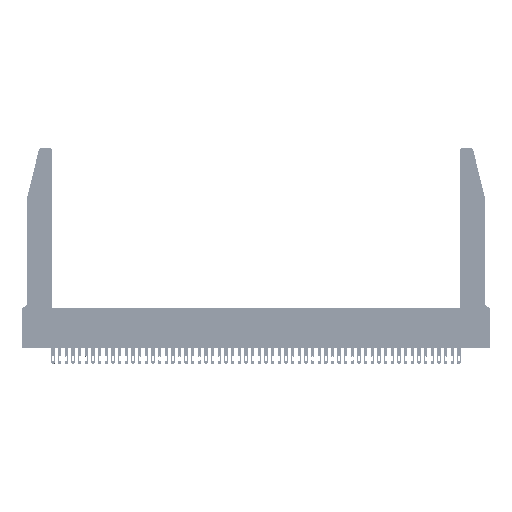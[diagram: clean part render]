
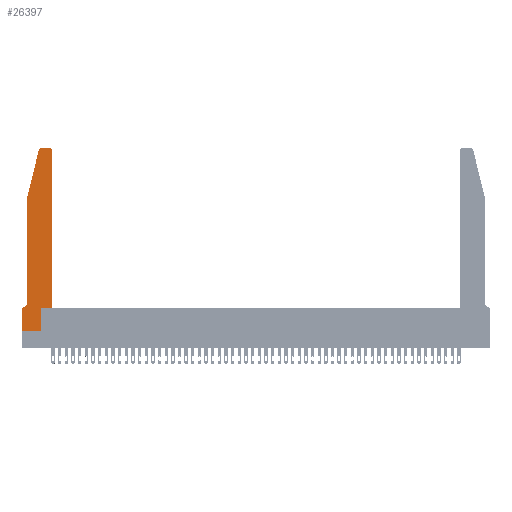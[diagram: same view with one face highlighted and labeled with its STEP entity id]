
A CAD part, top view. The second image highlights one B-rep face of the part: STEP entity #26397.
In plain terms, the highlighted planar face has unit normal (0, 0, 1).
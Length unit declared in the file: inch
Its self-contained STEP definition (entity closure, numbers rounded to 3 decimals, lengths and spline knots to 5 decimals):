
#550 = DIRECTION ( 'NONE',  ( -1., 0., 0. ) ) ;
#915 = CARTESIAN_POINT ( 'NONE',  ( 0.4505, 0.35, 0.37 ) ) ;
#1173 = VECTOR ( 'NONE', #18549, 39.37008 ) ;
#1265 = LINE ( 'NONE', #35917, #48980 ) ;
#2085 = AXIS2_PLACEMENT_3D ( 'NONE', #5946, #13271, #40658 ) ;
#2260 = ORIENTED_EDGE ( 'NONE', *, *, #8568, .T. ) ;
#3101 = DIRECTION ( 'NONE',  ( 1., 0., 0. ) ) ;
#3153 = EDGE_CURVE ( 'NONE', #23213, #50517, #5356, .T. ) ;
#3368 = CARTESIAN_POINT ( 'NONE',  ( 0., 0.35, 0.37 ) ) ;
#3682 = ORIENTED_EDGE ( 'NONE', *, *, #30100, .T. ) ;
#5268 = VECTOR ( 'NONE', #24191, 39.37008 ) ;
#5356 = LINE ( 'NONE', #44972, #32894 ) ;
#5617 = CARTESIAN_POINT ( 'NONE',  ( 0.4505, 0.35, 0.37 ) ) ;
#5848 = LINE ( 'NONE', #27617, #5268 ) ;
#5946 = CARTESIAN_POINT ( 'NONE',  ( 0.0055, 0.42, 0.37 ) ) ;
#6176 = VERTEX_POINT ( 'NONE', #3368 ) ;
#7727 = LINE ( 'NONE', #30731, #32263 ) ;
#8096 = CARTESIAN_POINT ( 'NONE',  ( 0.0755, 0.35, 0.37 ) ) ;
#8448 = EDGE_CURVE ( 'NONE', #16313, #36084, #45249, .T. ) ;
#8568 = EDGE_CURVE ( 'NONE', #17694, #30529, #43979, .T. ) ;
#8913 = ORIENTED_EDGE ( 'NONE', *, *, #10560, .T. ) ;
#8957 = AXIS2_PLACEMENT_3D ( 'NONE', #18659, #46000, #3101 ) ;
#9064 = ORIENTED_EDGE ( 'NONE', *, *, #30528, .T. ) ;
#9164 = LINE ( 'NONE', #34760, #10995 ) ;
#9933 = ORIENTED_EDGE ( 'NONE', *, *, #42092, .T. ) ;
#10155 = ORIENTED_EDGE ( 'NONE', *, *, #8448, .T. ) ;
#10560 = EDGE_CURVE ( 'NONE', #36084, #19034, #23695, .T. ) ;
#10995 = VECTOR ( 'NONE', #35103, 39.37008 ) ;
#11185 = FACE_OUTER_BOUND ( 'NONE', #21468, .T. ) ;
#11554 = VERTEX_POINT ( 'NONE', #20644 ) ;
#12856 = CARTESIAN_POINT ( 'NONE',  ( 0.25487, 2.72718, 0.37 ) ) ;
#12894 = CARTESIAN_POINT ( 'NONE',  ( 0.4205, 2.75, 0.37 ) ) ;
#13271 = DIRECTION ( 'NONE',  ( 0., 0., -1. ) ) ;
#13650 = CARTESIAN_POINT ( 'NONE',  ( 0.2865, 0.35, 0.37 ) ) ;
#14009 = EDGE_CURVE ( 'NONE', #11554, #17195, #1265, .T. ) ;
#14400 = ORIENTED_EDGE ( 'NONE', *, *, #14576, .T. ) ;
#14576 = EDGE_CURVE ( 'NONE', #17195, #17694, #9164, .T. ) ;
#14994 = ORIENTED_EDGE ( 'NONE', *, *, #14009, .T. ) ;
#15561 = VERTEX_POINT ( 'NONE', #39977 ) ;
#16313 = VERTEX_POINT ( 'NONE', #12894 ) ;
#16572 = DIRECTION ( 'NONE',  ( 0., 1., 0. ) ) ;
#16661 = DIRECTION ( 'NONE',  ( 0., 1., 0. ) ) ;
#17195 = VERTEX_POINT ( 'NONE', #13650 ) ;
#17450 = DIRECTION ( 'NONE',  ( 0., -1., 0. ) ) ;
#17694 = VERTEX_POINT ( 'NONE', #5617 ) ;
#17739 = DIRECTION ( 'NONE',  ( 1., 0., 0. ) ) ;
#18122 = AXIS2_PLACEMENT_3D ( 'NONE', #33801, #37242, #17739 ) ;
#18549 = DIRECTION ( 'NONE',  ( -1., 0., 0. ) ) ;
#18600 = CARTESIAN_POINT ( 'NONE',  ( 0.284, 2.75, 0.37 ) ) ;
#18659 = CARTESIAN_POINT ( 'NONE',  ( 0.4205, 2.72, 0.37 ) ) ;
#19034 = VERTEX_POINT ( 'NONE', #12856 ) ;
#20644 = CARTESIAN_POINT ( 'NONE',  ( 0.2865, 0., 0.37 ) ) ;
#21468 = EDGE_LOOP ( 'NONE', ( #10155, #8913, #9064, #26012, #30155, #9933, #26757, #3682, #14994, #14400, #2260, #50630 ) ) ;
#22279 = DIRECTION ( 'NONE',  ( 0., 0., 1. ) ) ;
#22285 = DIRECTION ( 'NONE',  ( 1., 0., 0. ) ) ;
#23201 = VECTOR ( 'NONE', #16661, 39.37008 ) ;
#23213 = VERTEX_POINT ( 'NONE', #44004 ) ;
#23695 = CIRCLE ( 'NONE', #18122, 0.03 ) ;
#24191 = DIRECTION ( 'NONE',  ( -0.239, -0.971, 0. ) ) ;
#26012 = ORIENTED_EDGE ( 'NONE', *, *, #3153, .T. ) ;
#26212 = DIRECTION ( 'NONE',  ( 1., 0., 0. ) ) ;
#26397 = ADVANCED_FACE ( 'NONE', ( #11185 ), #41935, .T. ) ;
#26757 = ORIENTED_EDGE ( 'NONE', *, *, #47592, .T. ) ;
#27617 = CARTESIAN_POINT ( 'NONE',  ( 0.0755, 2., 0.37 ) ) ;
#30100 = EDGE_CURVE ( 'NONE', #45808, #11554, #45047, .T. ) ;
#30155 = ORIENTED_EDGE ( 'NONE', *, *, #49687, .T. ) ;
#30528 = EDGE_CURVE ( 'NONE', #19034, #23213, #5848, .T. ) ;
#30529 = VERTEX_POINT ( 'NONE', #31538 ) ;
#30731 = CARTESIAN_POINT ( 'NONE',  ( 0., 0., 0.37 ) ) ;
#31538 = CARTESIAN_POINT ( 'NONE',  ( 0.4505, 2.72, 0.37 ) ) ;
#32263 = VECTOR ( 'NONE', #35010, 39.37008 ) ;
#32894 = VECTOR ( 'NONE', #17450, 39.37008 ) ;
#33801 = CARTESIAN_POINT ( 'NONE',  ( 0.284, 2.72, 0.37 ) ) ;
#34760 = CARTESIAN_POINT ( 'NONE',  ( 0.4505, 0.35, 0.37 ) ) ;
#35010 = DIRECTION ( 'NONE',  ( 0., -1., 0. ) ) ;
#35103 = DIRECTION ( 'NONE',  ( 1., 0., 0. ) ) ;
#35485 = CARTESIAN_POINT ( 'NONE',  ( 0.2605, 2.75, 0.37 ) ) ;
#35917 = CARTESIAN_POINT ( 'NONE',  ( 0.2865, 0.35, 0.37 ) ) ;
#36084 = VERTEX_POINT ( 'NONE', #18600 ) ;
#37242 = DIRECTION ( 'NONE',  ( 0., 0., 1. ) ) ;
#38132 = CIRCLE ( 'NONE', #2085, 0.07 ) ;
#38655 = CARTESIAN_POINT ( 'NONE',  ( 0., 0.35, 0.37 ) ) ;
#39465 = AXIS2_PLACEMENT_3D ( 'NONE', #38655, #22279, #26212 ) ;
#39977 = CARTESIAN_POINT ( 'NONE',  ( 0.0055, 0.35, 0.37 ) ) ;
#40399 = VECTOR ( 'NONE', #550, 39.37008 ) ;
#40658 = DIRECTION ( 'NONE',  ( -1., 0., 0. ) ) ;
#40732 = CARTESIAN_POINT ( 'NONE',  ( 0., 0., 0.37 ) ) ;
#41381 = VECTOR ( 'NONE', #22285, 39.37008 ) ;
#41935 = PLANE ( 'NONE',  #39465 ) ;
#42092 = EDGE_CURVE ( 'NONE', #15561, #6176, #47092, .T. ) ;
#42493 = CARTESIAN_POINT ( 'NONE',  ( 0.0755, 0.42, 0.37 ) ) ;
#43979 = LINE ( 'NONE', #915, #23201 ) ;
#44004 = CARTESIAN_POINT ( 'NONE',  ( 0.0755, 2., 0.37 ) ) ;
#44972 = CARTESIAN_POINT ( 'NONE',  ( 0.0755, 2., 0.37 ) ) ;
#45047 = LINE ( 'NONE', #49456, #41381 ) ;
#45249 = LINE ( 'NONE', #35485, #1173 ) ;
#45808 = VERTEX_POINT ( 'NONE', #40732 ) ;
#46000 = DIRECTION ( 'NONE',  ( 0., 0., 1. ) ) ;
#47092 = LINE ( 'NONE', #8096, #40399 ) ;
#47384 = CIRCLE ( 'NONE', #8957, 0.03 ) ;
#47592 = EDGE_CURVE ( 'NONE', #6176, #45808, #7727, .T. ) ;
#48932 = EDGE_CURVE ( 'NONE', #30529, #16313, #47384, .T. ) ;
#48980 = VECTOR ( 'NONE', #16572, 39.37008 ) ;
#49456 = CARTESIAN_POINT ( 'NONE',  ( 0., 0., 0.37 ) ) ;
#49687 = EDGE_CURVE ( 'NONE', #50517, #15561, #38132, .T. ) ;
#50517 = VERTEX_POINT ( 'NONE', #42493 ) ;
#50630 = ORIENTED_EDGE ( 'NONE', *, *, #48932, .T. ) ;
